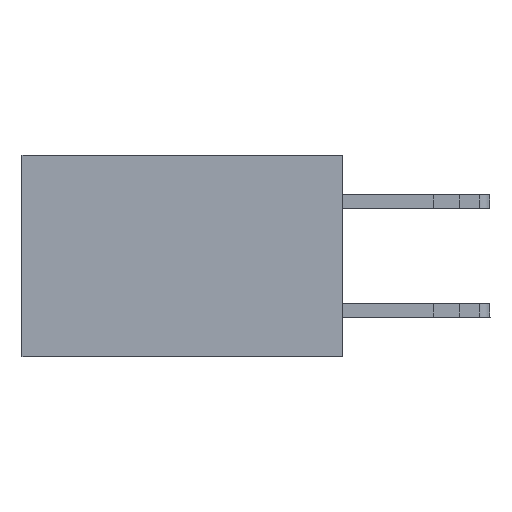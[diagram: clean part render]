
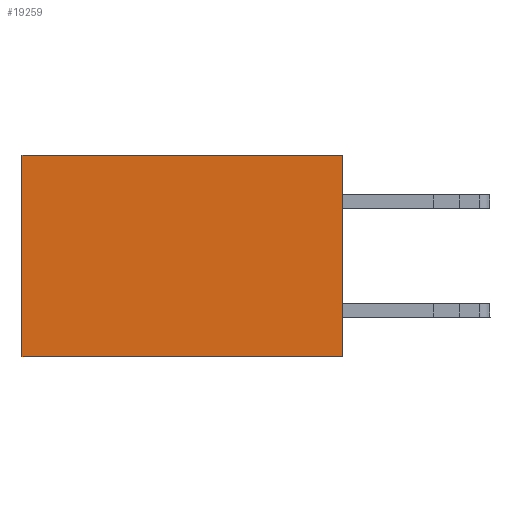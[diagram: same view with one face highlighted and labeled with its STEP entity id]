
A CAD part, left-side view. The second image highlights one B-rep face of the part: STEP entity #19259.
In plain terms, the highlighted planar face has unit normal (-1, 0, 0).
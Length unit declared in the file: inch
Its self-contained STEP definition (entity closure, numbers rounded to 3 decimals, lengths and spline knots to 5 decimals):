
#205 = VECTOR ( 'NONE', #14982, 39.37008 ) ;
#1007 = CARTESIAN_POINT ( 'NONE',  ( 0.277, 0., 0. ) ) ;
#2293 = CARTESIAN_POINT ( 'NONE',  ( 0.277, 0., -0.37 ) ) ;
#2633 = PLANE ( 'NONE',  #9193 ) ;
#4532 = VERTEX_POINT ( 'NONE', #22483 ) ;
#4738 = LINE ( 'NONE', #26697, #28405 ) ;
#5275 = DIRECTION ( 'NONE',  ( 0., 0., -1. ) ) ;
#6075 = EDGE_CURVE ( 'NONE', #19169, #4532, #4738, .T. ) ;
#6980 = DIRECTION ( 'NONE',  ( 0., 0., -1. ) ) ;
#9193 = AXIS2_PLACEMENT_3D ( 'NONE', #9695, #25668, #12078 ) ;
#9695 = CARTESIAN_POINT ( 'NONE',  ( 0.277, 0., -0.37 ) ) ;
#10264 = VERTEX_POINT ( 'NONE', #25201 ) ;
#12078 = DIRECTION ( 'NONE',  ( 0., 0., -1. ) ) ;
#14071 = EDGE_CURVE ( 'NONE', #27801, #10264, #29255, .T. ) ;
#14982 = DIRECTION ( 'NONE',  ( 0., 1., 0. ) ) ;
#15367 = LINE ( 'NONE', #28134, #26686 ) ;
#18027 = CARTESIAN_POINT ( 'NONE',  ( 0.277, 0., 0. ) ) ;
#18095 = LINE ( 'NONE', #2293, #23426 ) ;
#19169 = VERTEX_POINT ( 'NONE', #25390 ) ;
#19259 = ADVANCED_FACE ( 'NONE', ( #26966 ), #2633, .F. ) ;
#19814 = EDGE_CURVE ( 'NONE', #27801, #19169, #18095, .T. ) ;
#21014 = ORIENTED_EDGE ( 'NONE', *, *, #25998, .T. ) ;
#22223 = ORIENTED_EDGE ( 'NONE', *, *, #19814, .F. ) ;
#22483 = CARTESIAN_POINT ( 'NONE',  ( 0.277, 0.59, -0.37 ) ) ;
#23339 = ORIENTED_EDGE ( 'NONE', *, *, #14071, .T. ) ;
#23426 = VECTOR ( 'NONE', #6980, 39.37008 ) ;
#25201 = CARTESIAN_POINT ( 'NONE',  ( 0.277, 0.59, 0. ) ) ;
#25260 = ORIENTED_EDGE ( 'NONE', *, *, #6075, .F. ) ;
#25390 = CARTESIAN_POINT ( 'NONE',  ( 0.277, 0., -0.37 ) ) ;
#25668 = DIRECTION ( 'NONE',  ( 1., 0., 0. ) ) ;
#25998 = EDGE_CURVE ( 'NONE', #10264, #4532, #15367, .T. ) ;
#26452 = DIRECTION ( 'NONE',  ( 0., 1., 0. ) ) ;
#26686 = VECTOR ( 'NONE', #5275, 39.37008 ) ;
#26697 = CARTESIAN_POINT ( 'NONE',  ( 0.277, 0., -0.37 ) ) ;
#26966 = FACE_OUTER_BOUND ( 'NONE', #28882, .T. ) ;
#27801 = VERTEX_POINT ( 'NONE', #18027 ) ;
#28134 = CARTESIAN_POINT ( 'NONE',  ( 0.277, 0.59, -0.37 ) ) ;
#28405 = VECTOR ( 'NONE', #26452, 39.37008 ) ;
#28882 = EDGE_LOOP ( 'NONE', ( #21014, #25260, #22223, #23339 ) ) ;
#29255 = LINE ( 'NONE', #1007, #205 ) ;
